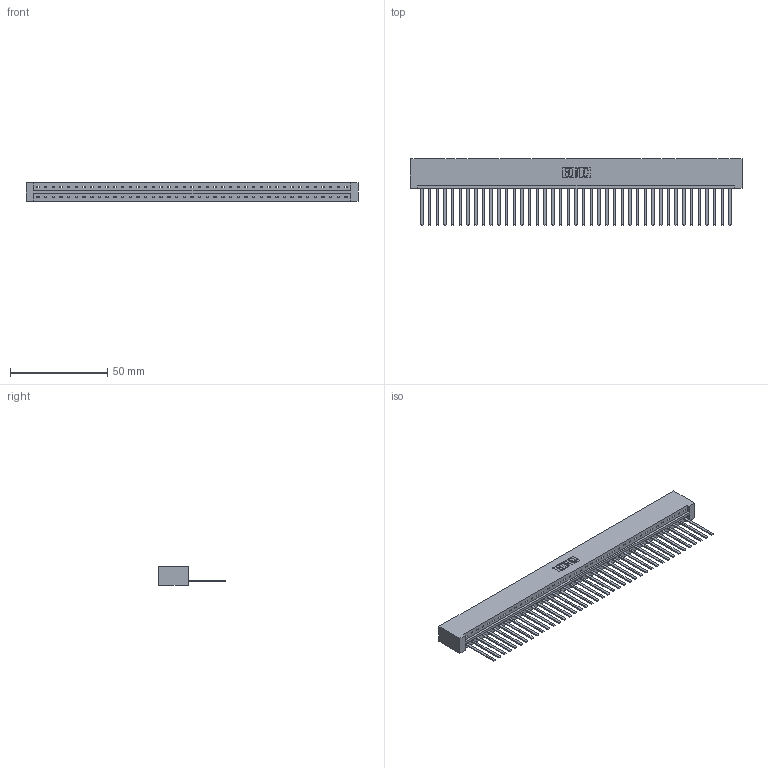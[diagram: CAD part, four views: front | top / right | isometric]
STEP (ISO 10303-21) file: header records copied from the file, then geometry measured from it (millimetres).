
FILE_DESCRIPTION (( 'STEP AP203' ), '1' );
FILE_NAME ('833-041-544-101.STEP', '2020-06-03T19:28:45', ( '' ), ( '' ), 'SwSTEP 2.0', 'SolidWorks 2020', '' );
FILE_SCHEMA (( 'CONFIG_CONTROL_DESIGN' ));
Length unit declared in the file: inch
Products named in the file (3): 833 Part_Lugless; 345-292-001_345-293-144; 833-041-544-101
Assembly tree (42 placements, depth 2):
  833-041-544-101
    833 Part_Lugless
    345-292-001_345-293-144  x41
Bounding box: 170.71 x 34.3 x 9.4 mm (x, y, z)
Volume: 18257.6 mm3; surface area: 21248.4 mm2
Topology: 42 solids, 42 shells, 2238 faces, 6765 edges, 4454 vertices
Faces by surface type: plane 1624, cylinder 614
Entity records: 24733 total; most frequent: CARTESIAN_POINT 4273, ORIENTED_EDGE 4250, DIRECTION 3595, EDGE_CURVE 2125, VECTOR 2009, LINE 2009, VERTEX_POINT 1414, AXIS2_PLACEMENT_3D 793
